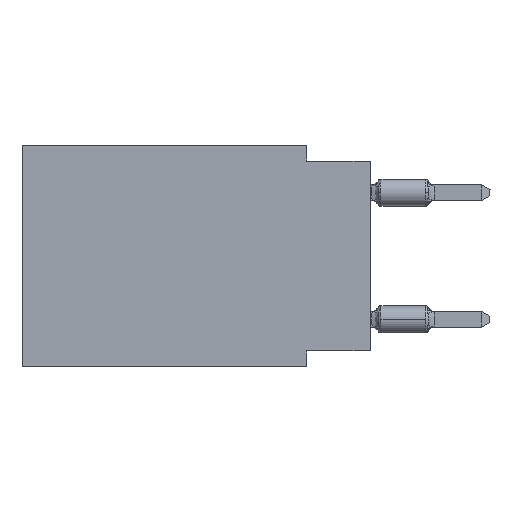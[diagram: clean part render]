
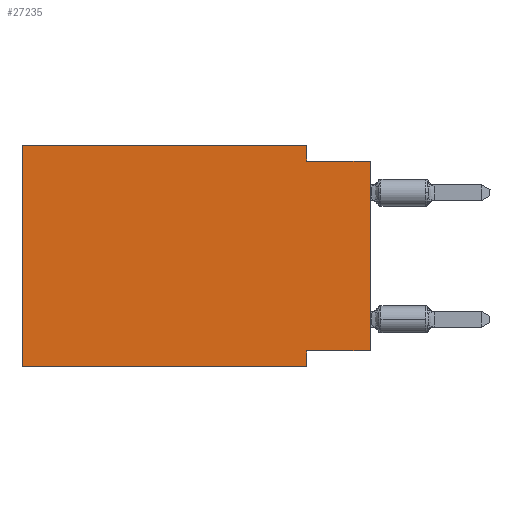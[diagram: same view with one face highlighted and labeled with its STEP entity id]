
A CAD part, left-side view. The second image highlights one B-rep face of the part: STEP entity #27235.
In plain terms, the highlighted planar face has unit normal (-1, 0, 0).
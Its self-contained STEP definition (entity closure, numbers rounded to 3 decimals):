
#369 = CARTESIAN_POINT ( 'NONE',  ( 0., 13.97, -8.89 ) ) ;
#2640 = ORIENTED_EDGE ( 'NONE', *, *, #17972, .F. ) ;
#3517 = DIRECTION ( 'NONE',  ( 0., 0., -1. ) ) ;
#3845 = CARTESIAN_POINT ( 'NONE',  ( 0., 2.54, 0. ) ) ;
#3950 = VERTEX_POINT ( 'NONE', #19556 ) ;
#4172 = ORIENTED_EDGE ( 'NONE', *, *, #33143, .F. ) ;
#4404 = VECTOR ( 'NONE', #39791, 1000. ) ;
#5626 = VERTEX_POINT ( 'NONE', #33572 ) ;
#5767 = EDGE_CURVE ( 'NONE', #24229, #23227, #51717, .T. ) ;
#5993 = CARTESIAN_POINT ( 'NONE',  ( 0., 2.54, -8.89 ) ) ;
#6327 = VERTEX_POINT ( 'NONE', #35081 ) ;
#6342 = DIRECTION ( 'NONE',  ( 1., 0., 0. ) ) ;
#7960 = LINE ( 'NONE', #17947, #19718 ) ;
#8469 = VECTOR ( 'NONE', #52539, 1000. ) ;
#8720 = EDGE_CURVE ( 'NONE', #53922, #24984, #50922, .T. ) ;
#11314 = PLANE ( 'NONE',  #20218 ) ;
#12904 = ORIENTED_EDGE ( 'NONE', *, *, #50180, .F. ) ;
#13941 = DIRECTION ( 'NONE',  ( 0., 1., 0. ) ) ;
#16638 = DIRECTION ( 'NONE',  ( 0., 0., -1. ) ) ;
#16971 = FACE_OUTER_BOUND ( 'NONE', #52712, .T. ) ;
#17698 = VECTOR ( 'NONE', #3517, 1000. ) ;
#17947 = CARTESIAN_POINT ( 'NONE',  ( 0., 0., -8.255 ) ) ;
#17972 = EDGE_CURVE ( 'NONE', #30533, #3950, #37357, .T. ) ;
#18408 = VECTOR ( 'NONE', #19688, 1000. ) ;
#19494 = ORIENTED_EDGE ( 'NONE', *, *, #63815, .F. ) ;
#19556 = CARTESIAN_POINT ( 'NONE',  ( 0., 2.54, 0. ) ) ;
#19688 = DIRECTION ( 'NONE',  ( 0., -1., 0. ) ) ;
#19718 = VECTOR ( 'NONE', #13941, 1000. ) ;
#20218 = AXIS2_PLACEMENT_3D ( 'NONE', #31608, #6342, #26619 ) ;
#23227 = VERTEX_POINT ( 'NONE', #37419 ) ;
#24229 = VERTEX_POINT ( 'NONE', #52717 ) ;
#24239 = ORIENTED_EDGE ( 'NONE', *, *, #39816, .F. ) ;
#24683 = CARTESIAN_POINT ( 'NONE',  ( 0., 2.54, -8.89 ) ) ;
#24984 = VERTEX_POINT ( 'NONE', #24683 ) ;
#26619 = DIRECTION ( 'NONE',  ( 0., 0., -1. ) ) ;
#26639 = ORIENTED_EDGE ( 'NONE', *, *, #5767, .T. ) ;
#26952 = LINE ( 'NONE', #37247, #8469 ) ;
#27235 = ADVANCED_FACE ( 'NONE', ( #16971 ), #11314, .F. ) ;
#27775 = VECTOR ( 'NONE', #61317, 1000. ) ;
#28048 = CARTESIAN_POINT ( 'NONE',  ( 0., 13.97, 0. ) ) ;
#29200 = CARTESIAN_POINT ( 'NONE',  ( 0., 13.97, 0. ) ) ;
#30533 = VERTEX_POINT ( 'NONE', #52419 ) ;
#30572 = VECTOR ( 'NONE', #16638, 1000. ) ;
#31608 = CARTESIAN_POINT ( 'NONE',  ( 0., 13.97, 0. ) ) ;
#32371 = DIRECTION ( 'NONE',  ( 0., -1., 0. ) ) ;
#32849 = VECTOR ( 'NONE', #32371, 1000. ) ;
#33143 = EDGE_CURVE ( 'NONE', #24229, #6327, #7960, .T. ) ;
#33572 = CARTESIAN_POINT ( 'NONE',  ( 0., 2.54, -0.635 ) ) ;
#35081 = CARTESIAN_POINT ( 'NONE',  ( 0., 2.54, -8.255 ) ) ;
#37247 = CARTESIAN_POINT ( 'NONE',  ( 0., 0., -0.635 ) ) ;
#37357 = LINE ( 'NONE', #28048, #32849 ) ;
#37419 = CARTESIAN_POINT ( 'NONE',  ( 0., 0., -0.635 ) ) ;
#38143 = ORIENTED_EDGE ( 'NONE', *, *, #8720, .T. ) ;
#39154 = LINE ( 'NONE', #29200, #4404 ) ;
#39791 = DIRECTION ( 'NONE',  ( 0., 0., 1. ) ) ;
#39816 = EDGE_CURVE ( 'NONE', #53922, #30533, #39154, .T. ) ;
#44654 = EDGE_CURVE ( 'NONE', #3950, #5626, #60620, .T. ) ;
#46552 = LINE ( 'NONE', #5993, #30572 ) ;
#50180 = EDGE_CURVE ( 'NONE', #5626, #23227, #26952, .T. ) ;
#50922 = LINE ( 'NONE', #369, #18408 ) ;
#51717 = LINE ( 'NONE', #61673, #27775 ) ;
#51791 = CARTESIAN_POINT ( 'NONE',  ( 0., 13.97, -8.89 ) ) ;
#52419 = CARTESIAN_POINT ( 'NONE',  ( 0., 13.97, 0. ) ) ;
#52539 = DIRECTION ( 'NONE',  ( 0., -1., 0. ) ) ;
#52712 = EDGE_LOOP ( 'NONE', ( #26639, #12904, #53500, #2640, #24239, #38143, #19494, #4172 ) ) ;
#52717 = CARTESIAN_POINT ( 'NONE',  ( 0., 0., -8.255 ) ) ;
#53500 = ORIENTED_EDGE ( 'NONE', *, *, #44654, .F. ) ;
#53922 = VERTEX_POINT ( 'NONE', #51791 ) ;
#60620 = LINE ( 'NONE', #3845, #17698 ) ;
#61317 = DIRECTION ( 'NONE',  ( 0., 0., 1. ) ) ;
#61673 = CARTESIAN_POINT ( 'NONE',  ( 0., 0., 0. ) ) ;
#63815 = EDGE_CURVE ( 'NONE', #6327, #24984, #46552, .T. ) ;
